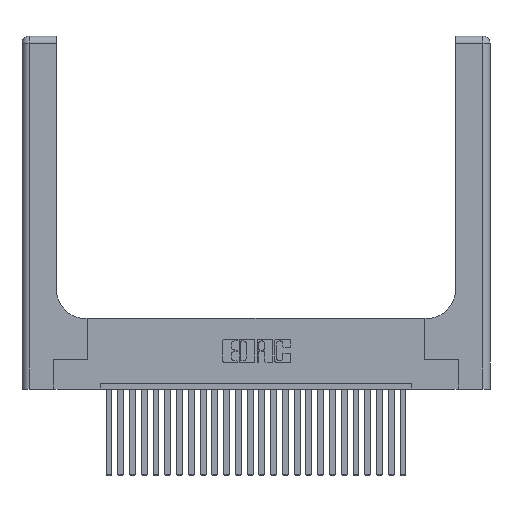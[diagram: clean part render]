
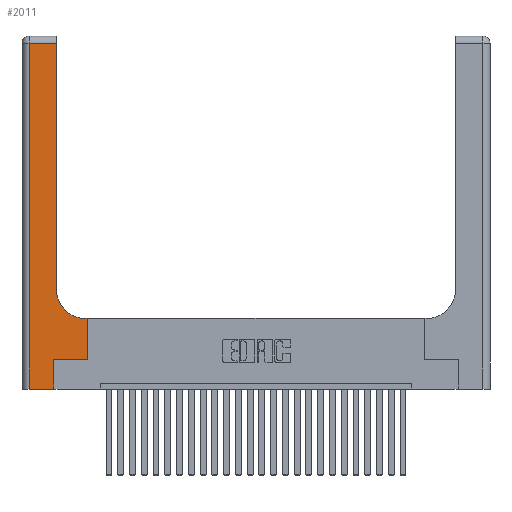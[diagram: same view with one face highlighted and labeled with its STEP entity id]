
A CAD part, top view. The second image highlights one B-rep face of the part: STEP entity #2011.
In plain terms, the highlighted planar face has unit normal (0, 0, 1).
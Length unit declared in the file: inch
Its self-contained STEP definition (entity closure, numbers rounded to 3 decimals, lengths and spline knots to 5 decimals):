
#859 = DIRECTION ( 'NONE',  ( 0., 1., 0. ) ) ;
#1816 = CARTESIAN_POINT ( 'NONE',  ( 0.5415, 0.6, 0.37 ) ) ;
#1963 = CARTESIAN_POINT ( 'NONE',  ( 0.269, 0.25, 0.37 ) ) ;
#1999 = DIRECTION ( 'NONE',  ( 0., -1., 0. ) ) ;
#2011 = ADVANCED_FACE ( 'NONE', ( #3771 ), #16362, .F. ) ;
#2286 = EDGE_CURVE ( 'NONE', #9773, #11946, #24725, .T. ) ;
#2449 = ORIENTED_EDGE ( 'NONE', *, *, #2286, .T. ) ;
#2456 = CARTESIAN_POINT ( 'NONE',  ( 0.5585, 0.6, 0.37 ) ) ;
#2677 = VECTOR ( 'NONE', #9149, 39.37008 ) ;
#2702 = CARTESIAN_POINT ( 'NONE',  ( 0.2915, 0.6, 0.37 ) ) ;
#2703 = ORIENTED_EDGE ( 'NONE', *, *, #4199, .T. ) ;
#2860 = CARTESIAN_POINT ( 'NONE',  ( 0., 0., 0.37 ) ) ;
#3192 = VECTOR ( 'NONE', #16279, 39.37008 ) ;
#3240 = CIRCLE ( 'NONE', #5320, 0.25 ) ;
#3289 = DIRECTION ( 'NONE',  ( 0., 1., 0. ) ) ;
#3490 = CARTESIAN_POINT ( 'NONE',  ( 0.2915, 2.94, 0.37 ) ) ;
#3544 = CARTESIAN_POINT ( 'NONE',  ( 0.269, 0.25, 0.37 ) ) ;
#3566 = ORIENTED_EDGE ( 'NONE', *, *, #11918, .T. ) ;
#3771 = FACE_OUTER_BOUND ( 'NONE', #20091, .T. ) ;
#4184 = ORIENTED_EDGE ( 'NONE', *, *, #26289, .T. ) ;
#4199 = EDGE_CURVE ( 'NONE', #10798, #4374, #24846, .T. ) ;
#4374 = VERTEX_POINT ( 'NONE', #3490 ) ;
#4669 = DIRECTION ( 'NONE',  ( 1., 0., 0. ) ) ;
#4776 = DIRECTION ( 'NONE',  ( -1., 0., 0. ) ) ;
#5320 = AXIS2_PLACEMENT_3D ( 'NONE', #15185, #17540, #17626 ) ;
#5974 = EDGE_CURVE ( 'NONE', #14785, #15447, #15071, .T. ) ;
#6029 = DIRECTION ( 'NONE',  ( 0., 0., -1. ) ) ;
#6045 = VECTOR ( 'NONE', #24075, 39.37008 ) ;
#7068 = CARTESIAN_POINT ( 'NONE',  ( 0.06, 2.94, 0.37 ) ) ;
#8544 = CARTESIAN_POINT ( 'NONE',  ( 0.06, 0., 0.37 ) ) ;
#8693 = ORIENTED_EDGE ( 'NONE', *, *, #14911, .T. ) ;
#8977 = CARTESIAN_POINT ( 'NONE',  ( 0., 2.94, 0.37 ) ) ;
#9061 = LINE ( 'NONE', #13092, #9404 ) ;
#9149 = DIRECTION ( 'NONE',  ( -1., 0., 0. ) ) ;
#9404 = VECTOR ( 'NONE', #3289, 39.37008 ) ;
#9773 = VERTEX_POINT ( 'NONE', #8544 ) ;
#9878 = EDGE_CURVE ( 'NONE', #4374, #23096, #24592, .T. ) ;
#10212 = LINE ( 'NONE', #3544, #6045 ) ;
#10798 = VERTEX_POINT ( 'NONE', #17142 ) ;
#11918 = EDGE_CURVE ( 'NONE', #15447, #15767, #23436, .T. ) ;
#11946 = VERTEX_POINT ( 'NONE', #16819 ) ;
#12128 = VECTOR ( 'NONE', #1999, 39.37008 ) ;
#12465 = LINE ( 'NONE', #18639, #12128 ) ;
#12561 = CARTESIAN_POINT ( 'NONE',  ( 0.5585, 0.25, 0.37 ) ) ;
#13092 = CARTESIAN_POINT ( 'NONE',  ( 0.269, 0., 0.37 ) ) ;
#14599 = VERTEX_POINT ( 'NONE', #1963 ) ;
#14785 = VERTEX_POINT ( 'NONE', #12561 ) ;
#14911 = EDGE_CURVE ( 'NONE', #11946, #14599, #9061, .T. ) ;
#15049 = ORIENTED_EDGE ( 'NONE', *, *, #5974, .T. ) ;
#15071 = LINE ( 'NONE', #24930, #3192 ) ;
#15185 = CARTESIAN_POINT ( 'NONE',  ( 0.5415, 0.85, 0.37 ) ) ;
#15447 = VERTEX_POINT ( 'NONE', #2456 ) ;
#15767 = VERTEX_POINT ( 'NONE', #1816 ) ;
#15991 = VECTOR ( 'NONE', #4669, 39.37008 ) ;
#16279 = DIRECTION ( 'NONE',  ( 0., 1., 0. ) ) ;
#16362 = PLANE ( 'NONE',  #21772 ) ;
#16819 = CARTESIAN_POINT ( 'NONE',  ( 0.269, 0., 0.37 ) ) ;
#16996 = ORIENTED_EDGE ( 'NONE', *, *, #26475, .T. ) ;
#17142 = CARTESIAN_POINT ( 'NONE',  ( 0.2915, 0.85, 0.37 ) ) ;
#17540 = DIRECTION ( 'NONE',  ( 0., 0., -1. ) ) ;
#17626 = DIRECTION ( 'NONE',  ( 1., 0., 0. ) ) ;
#18639 = CARTESIAN_POINT ( 'NONE',  ( 0.06, 3., 0.37 ) ) ;
#19246 = ORIENTED_EDGE ( 'NONE', *, *, #24860, .T. ) ;
#20091 = EDGE_LOOP ( 'NONE', ( #2703, #23633, #16996, #2449, #8693, #4184, #15049, #3566, #19246 ) ) ;
#20438 = DIRECTION ( 'NONE',  ( -1., 0., 0. ) ) ;
#21772 = AXIS2_PLACEMENT_3D ( 'NONE', #26480, #6029, #20438 ) ;
#22813 = VECTOR ( 'NONE', #4776, 39.37008 ) ;
#23096 = VERTEX_POINT ( 'NONE', #7068 ) ;
#23397 = CARTESIAN_POINT ( 'NONE',  ( 0.2915, 3., 0.37 ) ) ;
#23436 = LINE ( 'NONE', #2702, #22813 ) ;
#23633 = ORIENTED_EDGE ( 'NONE', *, *, #9878, .T. ) ;
#24075 = DIRECTION ( 'NONE',  ( 1., 0., 0. ) ) ;
#24221 = VECTOR ( 'NONE', #859, 39.37008 ) ;
#24592 = LINE ( 'NONE', #8977, #2677 ) ;
#24725 = LINE ( 'NONE', #2860, #15991 ) ;
#24846 = LINE ( 'NONE', #23397, #24221 ) ;
#24860 = EDGE_CURVE ( 'NONE', #15767, #10798, #3240, .T. ) ;
#24930 = CARTESIAN_POINT ( 'NONE',  ( 0.5585, 0.25, 0.37 ) ) ;
#26289 = EDGE_CURVE ( 'NONE', #14599, #14785, #10212, .T. ) ;
#26475 = EDGE_CURVE ( 'NONE', #23096, #9773, #12465, .T. ) ;
#26480 = CARTESIAN_POINT ( 'NONE',  ( 0., 3., 0.37 ) ) ;
